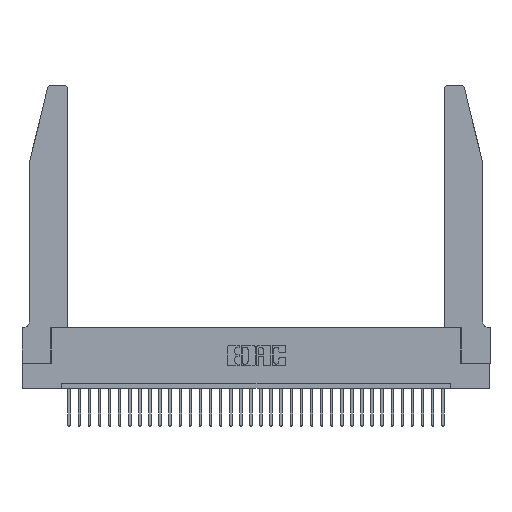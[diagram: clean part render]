
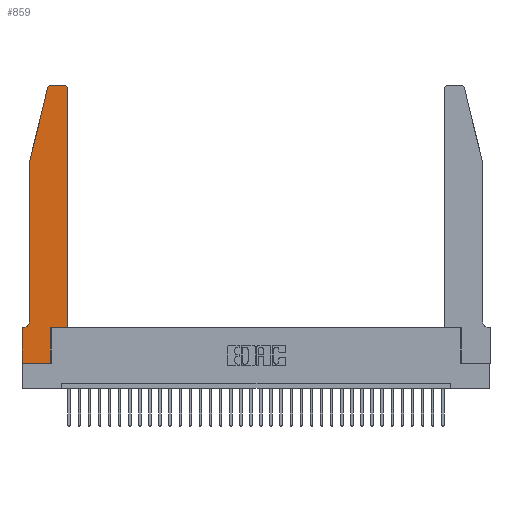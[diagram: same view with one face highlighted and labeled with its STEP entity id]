
A CAD part, top view. The second image highlights one B-rep face of the part: STEP entity #859.
In plain terms, the highlighted planar face has unit normal (0, 0, 1).
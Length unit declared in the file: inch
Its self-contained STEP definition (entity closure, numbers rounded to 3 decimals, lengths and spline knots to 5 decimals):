
#859 = ADVANCED_FACE ( 'NONE', ( #11645 ), #26442, .T. ) ;
#897 = DIRECTION ( 'NONE',  ( 1., 0., 0. ) ) ;
#1012 = CARTESIAN_POINT ( 'NONE',  ( 0.0755, 2., 0.37 ) ) ;
#2819 = LINE ( 'NONE', #10640, #29858 ) ;
#3411 = CARTESIAN_POINT ( 'NONE',  ( 0.4205, 2.72, 0.37 ) ) ;
#3705 = CARTESIAN_POINT ( 'NONE',  ( 0.0755, 2., 0.37 ) ) ;
#4126 = EDGE_CURVE ( 'NONE', #27963, #19210, #26034, .T. ) ;
#4522 = DIRECTION ( 'NONE',  ( 0., -1., 0. ) ) ;
#4785 = LINE ( 'NONE', #13204, #14288 ) ;
#5327 = LINE ( 'NONE', #8469, #33537 ) ;
#5337 = EDGE_CURVE ( 'NONE', #28786, #27963, #15785, .T. ) ;
#6419 = ORIENTED_EDGE ( 'NONE', *, *, #29111, .T. ) ;
#6705 = CARTESIAN_POINT ( 'NONE',  ( 0.2865, 0., 0.37 ) ) ;
#6737 = LINE ( 'NONE', #11571, #12981 ) ;
#7432 = AXIS2_PLACEMENT_3D ( 'NONE', #26223, #8148, #28827 ) ;
#7863 = ORIENTED_EDGE ( 'NONE', *, *, #19366, .T. ) ;
#7942 = EDGE_CURVE ( 'NONE', #10343, #17293, #2819, .T. ) ;
#8123 = CARTESIAN_POINT ( 'NONE',  ( 0.4505, 0.35, 0.37 ) ) ;
#8148 = DIRECTION ( 'NONE',  ( 0., 0., 1. ) ) ;
#8469 = CARTESIAN_POINT ( 'NONE',  ( 0.2605, 2.75, 0.37 ) ) ;
#8826 = ORIENTED_EDGE ( 'NONE', *, *, #5337, .T. ) ;
#9058 = DIRECTION ( 'NONE',  ( 1., 0., 0. ) ) ;
#9295 = VECTOR ( 'NONE', #18828, 39.37008 ) ;
#10343 = VERTEX_POINT ( 'NONE', #26175 ) ;
#10640 = CARTESIAN_POINT ( 'NONE',  ( 0., 0., 0.37 ) ) ;
#11090 = CARTESIAN_POINT ( 'NONE',  ( 0.4505, 2.72, 0.37 ) ) ;
#11571 = CARTESIAN_POINT ( 'NONE',  ( 0., 0., 0.37 ) ) ;
#11645 = FACE_OUTER_BOUND ( 'NONE', #29403, .T. ) ;
#12256 = CARTESIAN_POINT ( 'NONE',  ( 0.4205, 2.75, 0.37 ) ) ;
#12353 = CARTESIAN_POINT ( 'NONE',  ( 0.0055, 0.42, 0.37 ) ) ;
#12981 = VECTOR ( 'NONE', #32641, 39.37008 ) ;
#13085 = DIRECTION ( 'NONE',  ( -1., 0., 0. ) ) ;
#13204 = CARTESIAN_POINT ( 'NONE',  ( 0.4505, 0.35, 0.37 ) ) ;
#13780 = LINE ( 'NONE', #15285, #18230 ) ;
#14288 = VECTOR ( 'NONE', #9058, 39.37008 ) ;
#14900 = CARTESIAN_POINT ( 'NONE',  ( 0.0755, 2., 0.37 ) ) ;
#15285 = CARTESIAN_POINT ( 'NONE',  ( 0.2865, 0.35, 0.37 ) ) ;
#15377 = EDGE_CURVE ( 'NONE', #19210, #26391, #16253, .T. ) ;
#15437 = EDGE_CURVE ( 'NONE', #26391, #10343, #23977, .T. ) ;
#15539 = EDGE_CURVE ( 'NONE', #26879, #32688, #17449, .T. ) ;
#15785 = LINE ( 'NONE', #1012, #17435 ) ;
#16111 = ORIENTED_EDGE ( 'NONE', *, *, #33531, .T. ) ;
#16253 = CIRCLE ( 'NONE', #22521, 0.07 ) ;
#16492 = ORIENTED_EDGE ( 'NONE', *, *, #19536, .T. ) ;
#17106 = DIRECTION ( 'NONE',  ( -0.239, -0.971, 0. ) ) ;
#17293 = VERTEX_POINT ( 'NONE', #32793 ) ;
#17435 = VECTOR ( 'NONE', #17106, 39.37008 ) ;
#17449 = CIRCLE ( 'NONE', #29726, 0.03 ) ;
#17678 = DIRECTION ( 'NONE',  ( 0., 1., 0. ) ) ;
#17763 = DIRECTION ( 'NONE',  ( 0., 1., 0. ) ) ;
#17767 = EDGE_CURVE ( 'NONE', #29285, #19101, #4785, .T. ) ;
#18230 = VECTOR ( 'NONE', #17763, 39.37008 ) ;
#18488 = DIRECTION ( 'NONE',  ( -1., 0., 0. ) ) ;
#18749 = CARTESIAN_POINT ( 'NONE',  ( 0.25487, 2.72718, 0.37 ) ) ;
#18828 = DIRECTION ( 'NONE',  ( -1., 0., 0. ) ) ;
#19101 = VERTEX_POINT ( 'NONE', #8123 ) ;
#19210 = VERTEX_POINT ( 'NONE', #31673 ) ;
#19366 = EDGE_CURVE ( 'NONE', #17293, #32745, #6737, .T. ) ;
#19536 = EDGE_CURVE ( 'NONE', #32745, #29285, #13780, .T. ) ;
#19765 = DIRECTION ( 'NONE',  ( 1., 0., 0. ) ) ;
#20139 = ORIENTED_EDGE ( 'NONE', *, *, #4126, .T. ) ;
#20395 = ORIENTED_EDGE ( 'NONE', *, *, #15377, .T. ) ;
#20949 = DIRECTION ( 'NONE',  ( 0., -1., 0. ) ) ;
#21138 = CARTESIAN_POINT ( 'NONE',  ( 0.0055, 0.35, 0.37 ) ) ;
#22521 = AXIS2_PLACEMENT_3D ( 'NONE', #12353, #29176, #18488 ) ;
#22590 = EDGE_CURVE ( 'NONE', #32688, #26916, #5327, .T. ) ;
#22755 = VECTOR ( 'NONE', #4522, 39.37008 ) ;
#23440 = ORIENTED_EDGE ( 'NONE', *, *, #15539, .T. ) ;
#23977 = LINE ( 'NONE', #26350, #9295 ) ;
#24102 = AXIS2_PLACEMENT_3D ( 'NONE', #27005, #31161, #19765 ) ;
#25634 = ORIENTED_EDGE ( 'NONE', *, *, #7942, .T. ) ;
#26034 = LINE ( 'NONE', #14900, #22755 ) ;
#26175 = CARTESIAN_POINT ( 'NONE',  ( 0., 0.35, 0.37 ) ) ;
#26179 = VECTOR ( 'NONE', #17678, 39.37008 ) ;
#26223 = CARTESIAN_POINT ( 'NONE',  ( 0., 0.35, 0.37 ) ) ;
#26350 = CARTESIAN_POINT ( 'NONE',  ( 0.0755, 0.35, 0.37 ) ) ;
#26391 = VERTEX_POINT ( 'NONE', #21138 ) ;
#26442 = PLANE ( 'NONE',  #7432 ) ;
#26690 = DIRECTION ( 'NONE',  ( 0., 0., 1. ) ) ;
#26879 = VERTEX_POINT ( 'NONE', #11090 ) ;
#26916 = VERTEX_POINT ( 'NONE', #33543 ) ;
#27005 = CARTESIAN_POINT ( 'NONE',  ( 0.284, 2.72, 0.37 ) ) ;
#27814 = LINE ( 'NONE', #28173, #26179 ) ;
#27963 = VERTEX_POINT ( 'NONE', #3705 ) ;
#28173 = CARTESIAN_POINT ( 'NONE',  ( 0.4505, 0.35, 0.37 ) ) ;
#28556 = CARTESIAN_POINT ( 'NONE',  ( 0.2865, 0.35, 0.37 ) ) ;
#28786 = VERTEX_POINT ( 'NONE', #18749 ) ;
#28827 = DIRECTION ( 'NONE',  ( 1., 0., 0. ) ) ;
#29111 = EDGE_CURVE ( 'NONE', #26916, #28786, #32161, .T. ) ;
#29176 = DIRECTION ( 'NONE',  ( 0., 0., -1. ) ) ;
#29285 = VERTEX_POINT ( 'NONE', #28556 ) ;
#29403 = EDGE_LOOP ( 'NONE', ( #32787, #6419, #8826, #20139, #20395, #32782, #25634, #7863, #16492, #31355, #16111, #23440 ) ) ;
#29726 = AXIS2_PLACEMENT_3D ( 'NONE', #3411, #26690, #897 ) ;
#29858 = VECTOR ( 'NONE', #20949, 39.37008 ) ;
#31161 = DIRECTION ( 'NONE',  ( 0., 0., 1. ) ) ;
#31355 = ORIENTED_EDGE ( 'NONE', *, *, #17767, .T. ) ;
#31673 = CARTESIAN_POINT ( 'NONE',  ( 0.0755, 0.42, 0.37 ) ) ;
#32161 = CIRCLE ( 'NONE', #24102, 0.03 ) ;
#32641 = DIRECTION ( 'NONE',  ( 1., 0., 0. ) ) ;
#32688 = VERTEX_POINT ( 'NONE', #12256 ) ;
#32745 = VERTEX_POINT ( 'NONE', #6705 ) ;
#32782 = ORIENTED_EDGE ( 'NONE', *, *, #15437, .T. ) ;
#32787 = ORIENTED_EDGE ( 'NONE', *, *, #22590, .T. ) ;
#32793 = CARTESIAN_POINT ( 'NONE',  ( 0., 0., 0.37 ) ) ;
#33531 = EDGE_CURVE ( 'NONE', #19101, #26879, #27814, .T. ) ;
#33537 = VECTOR ( 'NONE', #13085, 39.37008 ) ;
#33543 = CARTESIAN_POINT ( 'NONE',  ( 0.284, 2.75, 0.37 ) ) ;
